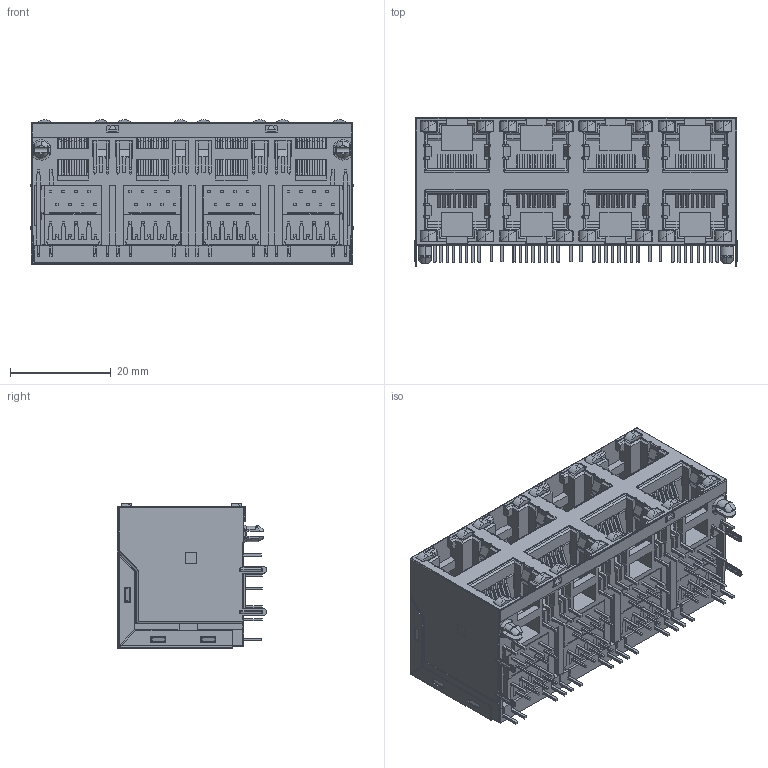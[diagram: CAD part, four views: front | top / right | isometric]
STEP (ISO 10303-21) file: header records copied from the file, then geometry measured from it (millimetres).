
FILE_DESCRIPTION (( 'STEP AP203' ), '1' );
FILE_NAME ('J96088892P88121.STEP', '2020-03-24T04:33:26', ( '' ), ( '' ), 'SwSTEP 2.0', 'SolidWorks 2016', '' );
FILE_SCHEMA (( 'CONFIG_CONTROL_DESIGN' ));
Length unit declared in the file: millimetre
Products named in the file (14): 96 Grounding_8 Ports; J96088892P88121; 96 Contact Lock Upper; 96 LED LH Upper_8-Red-Yellow; 96 LED RH Upper_8-Red-Yellow; 96 Contacts Lower; 96 Insulator_8 Ports; 96 Contact Lock Lower; 96 Insulator Insert; 96 LED LH Lower_8-Red-Yellow; 96 LED RH Lower_8-Red-Yellow; 96 Contacts Upper; 96 Shield_8 Ports LED - No EMI; 96 Back Plate_8 Ports
Assembly tree (40 placements, depth 2):
  J96088892P88121
    96 Insulator_8 Ports
    96 LED LH Lower_8-Red-Yellow  x4
    96 LED RH Lower_8-Red-Yellow  x4
    96 Contacts Lower  x4
    96 Contact Lock Lower  x4
    96 Grounding_8 Ports
    96 Contacts Upper  x4
    96 Contact Lock Upper  x4
    96 Insulator Insert  x4
    96 LED LH Upper_8-Red-Yellow  x4
    96 LED RH Upper_8-Red-Yellow  x4
    96 Back Plate_8 Ports
    96 Shield_8 Ports LED - No EMI
Bounding box: 64.05 x 29.58 x 28.68 mm (x, y, z)
Volume: 24160 mm3; surface area: 63657.9 mm2
Topology: 96 solids, 96 shells, 7674 faces, 21526 edges, 13818 vertices
Faces by surface type: plane 6069, cylinder 1339, bspline 252, cone 14
Entity records: 143174 total; most frequent: CARTESIAN_POINT 31548, ORIENTED_EDGE 24372, DIRECTION 20483, EDGE_CURVE 12186, LINE 9971, VECTOR 9971, VERTEX_POINT 7873, AXIS2_PLACEMENT_3D 5256
